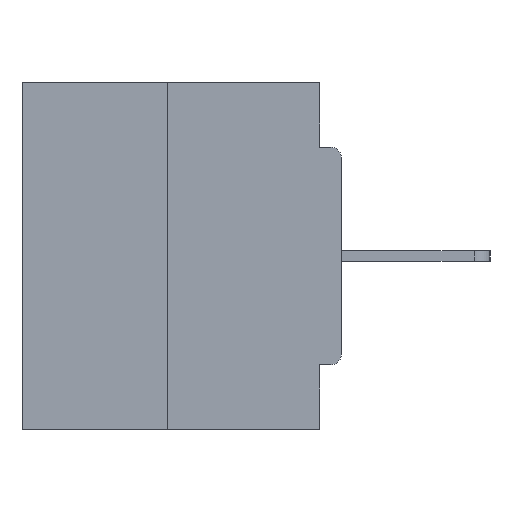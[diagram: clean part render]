
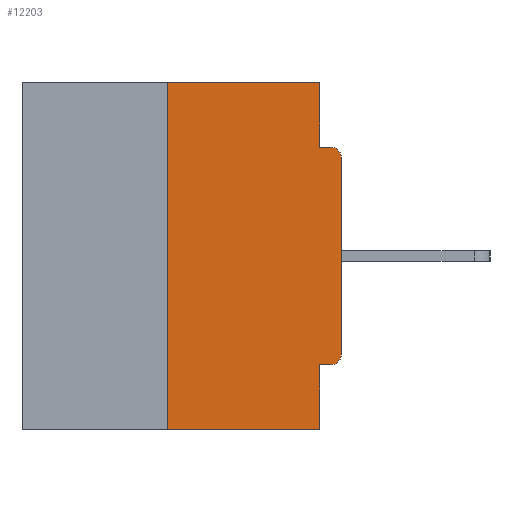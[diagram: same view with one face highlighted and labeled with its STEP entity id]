
A CAD part, left-side view. The second image highlights one B-rep face of the part: STEP entity #12203.
In plain terms, the highlighted planar face has unit normal (-1, 0, 0).
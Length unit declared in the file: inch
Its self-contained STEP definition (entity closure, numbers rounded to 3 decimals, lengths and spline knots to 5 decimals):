
#15 = DIRECTION ( 'NONE',  ( 0., 0., 1. ) ) ;
#76 = EDGE_CURVE ( 'NONE', #9613, #5361, #14742, .T. ) ;
#159 = DIRECTION ( 'NONE',  ( 0., 0., -1. ) ) ;
#212 = EDGE_LOOP ( 'NONE', ( #16723, #17134, #23603, #27280, #28037, #17706, #17793, #23773, #19558, #18494 ) ) ;
#274 = VECTOR ( 'NONE', #159, 39.37008 ) ;
#685 = VERTEX_POINT ( 'NONE', #6490 ) ;
#699 = CARTESIAN_POINT ( 'NONE',  ( 0., 0.031, -0.4065 ) ) ;
#750 = DIRECTION ( 'NONE',  ( 0., -1., 0. ) ) ;
#1370 = CARTESIAN_POINT ( 'NONE',  ( 0., 0.46, 0. ) ) ;
#2203 = VERTEX_POINT ( 'NONE', #6113 ) ;
#2310 = CARTESIAN_POINT ( 'NONE',  ( 0., 0.25, 0. ) ) ;
#2571 = CARTESIAN_POINT ( 'NONE',  ( 0., 0., -0.4065 ) ) ;
#2735 = VECTOR ( 'NONE', #24450, 39.37008 ) ;
#3067 = CARTESIAN_POINT ( 'NONE',  ( 0., 0., -0.0935 ) ) ;
#3214 = VECTOR ( 'NONE', #21284, 39.37008 ) ;
#3367 = LINE ( 'NONE', #11390, #14673 ) ;
#3548 = VECTOR ( 'NONE', #21702, 39.37008 ) ;
#3638 = EDGE_CURVE ( 'NONE', #9613, #25052, #20470, .T. ) ;
#3687 = EDGE_CURVE ( 'NONE', #28205, #11294, #25665, .T. ) ;
#5361 = VERTEX_POINT ( 'NONE', #699 ) ;
#5960 = DIRECTION ( 'NONE',  ( 0., 0., -1. ) ) ;
#6002 = CARTESIAN_POINT ( 'NONE',  ( 0., 0.031, -0.5 ) ) ;
#6006 = LINE ( 'NONE', #20140, #18630 ) ;
#6113 = CARTESIAN_POINT ( 'NONE',  ( 0., 0., -0.1085 ) ) ;
#6384 = EDGE_CURVE ( 'NONE', #28205, #24666, #6006, .T. ) ;
#6490 = CARTESIAN_POINT ( 'NONE',  ( 0., 0.015, -0.0935 ) ) ;
#6747 = CARTESIAN_POINT ( 'NONE',  ( 0., 0.015, -0.4065 ) ) ;
#6919 = CARTESIAN_POINT ( 'NONE',  ( 0., 0.031, -0.5 ) ) ;
#8052 = VERTEX_POINT ( 'NONE', #25396 ) ;
#9580 = LINE ( 'NONE', #6002, #3548 ) ;
#9613 = VERTEX_POINT ( 'NONE', #6747 ) ;
#10278 = LINE ( 'NONE', #3067, #26641 ) ;
#10804 = CARTESIAN_POINT ( 'NONE',  ( 0., 0.015, -0.1085 ) ) ;
#10972 = CARTESIAN_POINT ( 'NONE',  ( 0., 0.031, 0. ) ) ;
#11294 = VERTEX_POINT ( 'NONE', #2310 ) ;
#11390 = CARTESIAN_POINT ( 'NONE',  ( 0., 0., 0. ) ) ;
#12041 = CARTESIAN_POINT ( 'NONE',  ( 0., 0.25, -0.5 ) ) ;
#12203 = ADVANCED_FACE ( 'NONE', ( #26037 ), #17116, .F. ) ;
#12287 = EDGE_CURVE ( 'NONE', #2203, #685, #23971, .T. ) ;
#13083 = DIRECTION ( 'NONE',  ( 0., 0., -1. ) ) ;
#13169 = VECTOR ( 'NONE', #27189, 39.37008 ) ;
#14148 = EDGE_CURVE ( 'NONE', #8052, #685, #10278, .T. ) ;
#14673 = VECTOR ( 'NONE', #15, 39.37008 ) ;
#14742 = LINE ( 'NONE', #2571, #2735 ) ;
#15156 = CARTESIAN_POINT ( 'NONE',  ( 0., 0., -0.3915 ) ) ;
#15981 = CARTESIAN_POINT ( 'NONE',  ( 0., 0.031, 0. ) ) ;
#16553 = EDGE_CURVE ( 'NONE', #5361, #24666, #9580, .T. ) ;
#16589 = LINE ( 'NONE', #23411, #3214 ) ;
#16723 = ORIENTED_EDGE ( 'NONE', *, *, #22946, .F. ) ;
#17116 = PLANE ( 'NONE',  #27105 ) ;
#17134 = ORIENTED_EDGE ( 'NONE', *, *, #3687, .F. ) ;
#17706 = ORIENTED_EDGE ( 'NONE', *, *, #3638, .T. ) ;
#17793 = ORIENTED_EDGE ( 'NONE', *, *, #26485, .T. ) ;
#17963 = VERTEX_POINT ( 'NONE', #10972 ) ;
#18494 = ORIENTED_EDGE ( 'NONE', *, *, #28695, .F. ) ;
#18630 = VECTOR ( 'NONE', #19850, 39.37008 ) ;
#19409 = DIRECTION ( 'NONE',  ( 1., 0., 0. ) ) ;
#19558 = ORIENTED_EDGE ( 'NONE', *, *, #14148, .F. ) ;
#19850 = DIRECTION ( 'NONE',  ( 0., -1., 0. ) ) ;
#20140 = CARTESIAN_POINT ( 'NONE',  ( 0., 0.46, -0.5 ) ) ;
#20470 = CIRCLE ( 'NONE', #22886, 0.015 ) ;
#21284 = DIRECTION ( 'NONE',  ( 0., -1., 0. ) ) ;
#21702 = DIRECTION ( 'NONE',  ( 0., 0., -1. ) ) ;
#22886 = AXIS2_PLACEMENT_3D ( 'NONE', #27989, #27959, #27954 ) ;
#22946 = EDGE_CURVE ( 'NONE', #11294, #17963, #16589, .T. ) ;
#23411 = CARTESIAN_POINT ( 'NONE',  ( 0., 0.46, 0. ) ) ;
#23529 = LINE ( 'NONE', #15981, #274 ) ;
#23603 = ORIENTED_EDGE ( 'NONE', *, *, #6384, .T. ) ;
#23773 = ORIENTED_EDGE ( 'NONE', *, *, #12287, .T. ) ;
#23971 = CIRCLE ( 'NONE', #25620, 0.015 ) ;
#24450 = DIRECTION ( 'NONE',  ( 0., 1., 0. ) ) ;
#24666 = VERTEX_POINT ( 'NONE', #6919 ) ;
#25052 = VERTEX_POINT ( 'NONE', #15156 ) ;
#25396 = CARTESIAN_POINT ( 'NONE',  ( 0., 0.031, -0.0935 ) ) ;
#25620 = AXIS2_PLACEMENT_3D ( 'NONE', #10804, #26362, #13083 ) ;
#25665 = LINE ( 'NONE', #26934, #13169 ) ;
#26037 = FACE_OUTER_BOUND ( 'NONE', #212, .T. ) ;
#26362 = DIRECTION ( 'NONE',  ( -1., 0., 0. ) ) ;
#26485 = EDGE_CURVE ( 'NONE', #25052, #2203, #3367, .T. ) ;
#26641 = VECTOR ( 'NONE', #750, 39.37008 ) ;
#26934 = CARTESIAN_POINT ( 'NONE',  ( 0., 0.25, 0. ) ) ;
#27105 = AXIS2_PLACEMENT_3D ( 'NONE', #1370, #19409, #5960 ) ;
#27189 = DIRECTION ( 'NONE',  ( 0., 0., 1. ) ) ;
#27280 = ORIENTED_EDGE ( 'NONE', *, *, #16553, .F. ) ;
#27954 = DIRECTION ( 'NONE',  ( 0., 0., -1. ) ) ;
#27959 = DIRECTION ( 'NONE',  ( -1., 0., 0. ) ) ;
#27989 = CARTESIAN_POINT ( 'NONE',  ( 0., 0.015, -0.3915 ) ) ;
#28037 = ORIENTED_EDGE ( 'NONE', *, *, #76, .F. ) ;
#28205 = VERTEX_POINT ( 'NONE', #12041 ) ;
#28695 = EDGE_CURVE ( 'NONE', #17963, #8052, #23529, .T. ) ;
